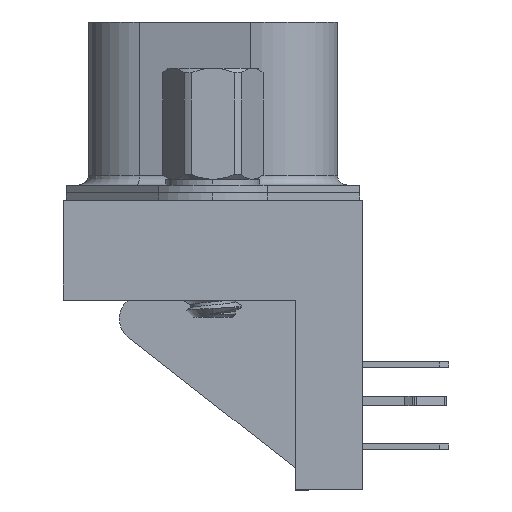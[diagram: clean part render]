
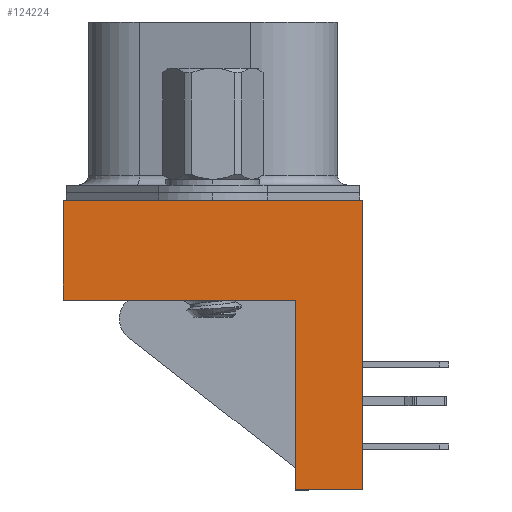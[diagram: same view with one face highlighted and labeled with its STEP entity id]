
A CAD part, left-side view. The second image highlights one B-rep face of the part: STEP entity #124224.
In plain terms, the highlighted planar face has unit normal (-1, 0, 0).
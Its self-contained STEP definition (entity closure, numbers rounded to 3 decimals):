
#1405 = CARTESIAN_POINT ( 'NONE',  ( -4.125, -7.8, -15.1 ) ) ;
#2591 = ORIENTED_EDGE ( 'NONE', *, *, #146402, .F. ) ;
#2605 = CARTESIAN_POINT ( 'NONE',  ( -4.125, 7.8, -15.1 ) ) ;
#5300 = VECTOR ( 'NONE', #50189, 1000. ) ;
#8961 = CARTESIAN_POINT ( 'NONE',  ( -4.125, -7.8, 0. ) ) ;
#10312 = CARTESIAN_POINT ( 'NONE',  ( -4.125, 7.8, 0. ) ) ;
#15985 = VERTEX_POINT ( 'NONE', #8961 ) ;
#23127 = CARTESIAN_POINT ( 'NONE',  ( -4.125, -4.3, -15.1 ) ) ;
#27683 = DIRECTION ( 'NONE',  ( 0., -1., 0. ) ) ;
#28873 = EDGE_CURVE ( 'NONE', #166037, #39181, #171542, .T. ) ;
#32450 = DIRECTION ( 'NONE',  ( 0., 0., 1. ) ) ;
#33095 = PLANE ( 'NONE',  #155565 ) ;
#35369 = LINE ( 'NONE', #95032, #58031 ) ;
#39181 = VERTEX_POINT ( 'NONE', #82681 ) ;
#45231 = DIRECTION ( 'NONE',  ( 0., -1., 0. ) ) ;
#48340 = CARTESIAN_POINT ( 'NONE',  ( -4.125, 7.8, -5.2 ) ) ;
#48779 = ORIENTED_EDGE ( 'NONE', *, *, #77243, .F. ) ;
#50189 = DIRECTION ( 'NONE',  ( 0., 0., 1. ) ) ;
#51679 = EDGE_LOOP ( 'NONE', ( #48779, #2591, #162144, #109270, #67647, #152249 ) ) ;
#58031 = VECTOR ( 'NONE', #79193, 1000. ) ;
#67647 = ORIENTED_EDGE ( 'NONE', *, *, #121912, .F. ) ;
#68795 = VERTEX_POINT ( 'NONE', #178169 ) ;
#77243 = EDGE_CURVE ( 'NONE', #143050, #166037, #104326, .T. ) ;
#79193 = DIRECTION ( 'NONE',  ( 0., 0., 1. ) ) ;
#79413 = EDGE_CURVE ( 'NONE', #89798, #15985, #35369, .T. ) ;
#82681 = CARTESIAN_POINT ( 'NONE',  ( -4.125, 7.8, 0. ) ) ;
#83941 = CARTESIAN_POINT ( 'NONE',  ( -4.125, -4.3, -5.2 ) ) ;
#87292 = CARTESIAN_POINT ( 'NONE',  ( -4.125, 7.8, -5.2 ) ) ;
#88146 = DIRECTION ( 'NONE',  ( -1., 0., 0. ) ) ;
#89798 = VERTEX_POINT ( 'NONE', #1405 ) ;
#92557 = VECTOR ( 'NONE', #27683, 1000. ) ;
#93131 = LINE ( 'NONE', #23127, #5300 ) ;
#95032 = CARTESIAN_POINT ( 'NONE',  ( -4.125, -7.8, -15.1 ) ) ;
#100904 = EDGE_CURVE ( 'NONE', #68795, #89798, #169522, .T. ) ;
#104326 = LINE ( 'NONE', #48340, #173205 ) ;
#105247 = DIRECTION ( 'NONE',  ( 0., 1., 0. ) ) ;
#109208 = DIRECTION ( 'NONE',  ( 0., -1., 0. ) ) ;
#109270 = ORIENTED_EDGE ( 'NONE', *, *, #79413, .T. ) ;
#121912 = EDGE_CURVE ( 'NONE', #39181, #15985, #139063, .T. ) ;
#124224 = ADVANCED_FACE ( 'NONE', ( #158153 ), #33095, .T. ) ;
#137191 = VECTOR ( 'NONE', #109208, 1000. ) ;
#139003 = VECTOR ( 'NONE', #32450, 1000. ) ;
#139063 = LINE ( 'NONE', #10312, #137191 ) ;
#143050 = VERTEX_POINT ( 'NONE', #83941 ) ;
#146402 = EDGE_CURVE ( 'NONE', #68795, #143050, #93131, .T. ) ;
#152249 = ORIENTED_EDGE ( 'NONE', *, *, #28873, .F. ) ;
#155520 = CARTESIAN_POINT ( 'NONE',  ( -4.125, 7.8, -15.1 ) ) ;
#155565 = AXIS2_PLACEMENT_3D ( 'NONE', #172160, #88146, #45231 ) ;
#158153 = FACE_OUTER_BOUND ( 'NONE', #51679, .T. ) ;
#162144 = ORIENTED_EDGE ( 'NONE', *, *, #100904, .T. ) ;
#166037 = VERTEX_POINT ( 'NONE', #87292 ) ;
#169522 = LINE ( 'NONE', #155520, #92557 ) ;
#171542 = LINE ( 'NONE', #2605, #139003 ) ;
#172160 = CARTESIAN_POINT ( 'NONE',  ( -4.125, 7.8, -15.1 ) ) ;
#173205 = VECTOR ( 'NONE', #105247, 1000. ) ;
#178169 = CARTESIAN_POINT ( 'NONE',  ( -4.125, -4.3, -15.1 ) ) ;
